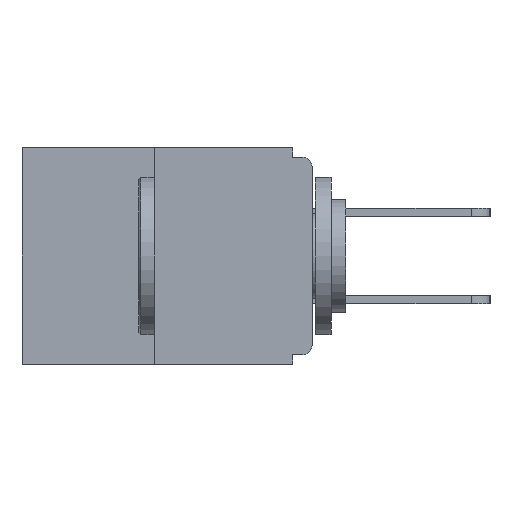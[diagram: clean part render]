
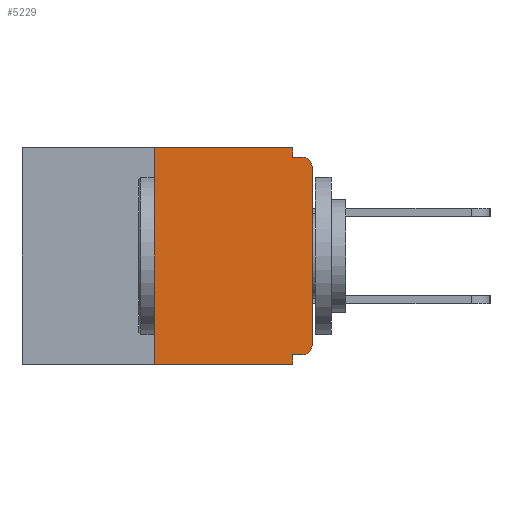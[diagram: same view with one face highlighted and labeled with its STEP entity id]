
A CAD part, left-side view. The second image highlights one B-rep face of the part: STEP entity #5229.
In plain terms, the highlighted planar face has unit normal (-1, 0, 0).
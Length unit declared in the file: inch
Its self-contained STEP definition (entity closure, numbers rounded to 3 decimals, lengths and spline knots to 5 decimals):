
#596 = AXIS2_PLACEMENT_3D ( 'NONE', #19665, #8271, #16163 ) ;
#840 = DIRECTION ( 'NONE',  ( 0., 0., -1. ) ) ;
#916 = ORIENTED_EDGE ( 'NONE', *, *, #10833, .F. ) ;
#1297 = DIRECTION ( 'NONE',  ( 0., 0., 1. ) ) ;
#1313 = PLANE ( 'NONE',  #23732 ) ;
#1740 = CARTESIAN_POINT ( 'NONE',  ( 0., 0., -0.328 ) ) ;
#2377 = FACE_OUTER_BOUND ( 'NONE', #3800, .T. ) ;
#2539 = DIRECTION ( 'NONE',  ( 0., 0., 1. ) ) ;
#3269 = CARTESIAN_POINT ( 'NONE',  ( 0., 0., -0.313 ) ) ;
#3676 = DIRECTION ( 'NONE',  ( 0., 0., -1. ) ) ;
#3800 = EDGE_LOOP ( 'NONE', ( #14801, #8469, #24225, #5966, #916, #23715, #18617, #8338, #15374, #19220 ) ) ;
#3841 = EDGE_CURVE ( 'NONE', #18358, #21685, #25170, .T. ) ;
#5088 = EDGE_CURVE ( 'NONE', #18833, #5514, #5436, .T. ) ;
#5229 = ADVANCED_FACE ( 'NONE', ( #2377 ), #1313, .F. ) ;
#5434 = CARTESIAN_POINT ( 'NONE',  ( 0., 0.015, -0.328 ) ) ;
#5436 = LINE ( 'NONE', #8785, #19596 ) ;
#5514 = VERTEX_POINT ( 'NONE', #10177 ) ;
#5833 = CARTESIAN_POINT ( 'NONE',  ( 0., 0.015, -0.03 ) ) ;
#5950 = VECTOR ( 'NONE', #2539, 39.37008 ) ;
#5966 = ORIENTED_EDGE ( 'NONE', *, *, #5088, .F. ) ;
#6164 = CARTESIAN_POINT ( 'NONE',  ( 0., 0.031, 0. ) ) ;
#6411 = CARTESIAN_POINT ( 'NONE',  ( 0., 0.015, -0.015 ) ) ;
#6547 = DIRECTION ( 'NONE',  ( 0., -1., 0. ) ) ;
#6632 = AXIS2_PLACEMENT_3D ( 'NONE', #5833, #23604, #3676 ) ;
#6744 = EDGE_CURVE ( 'NONE', #7429, #5514, #15855, .T. ) ;
#6960 = DIRECTION ( 'NONE',  ( 1., 0., 0. ) ) ;
#7358 = EDGE_CURVE ( 'NONE', #16632, #21954, #15472, .T. ) ;
#7429 = VERTEX_POINT ( 'NONE', #8364 ) ;
#8271 = DIRECTION ( 'NONE',  ( -1., 0., 0. ) ) ;
#8338 = ORIENTED_EDGE ( 'NONE', *, *, #22774, .T. ) ;
#8364 = CARTESIAN_POINT ( 'NONE',  ( 0., 0.25, -0.343 ) ) ;
#8469 = ORIENTED_EDGE ( 'NONE', *, *, #19182, .F. ) ;
#8528 = CARTESIAN_POINT ( 'NONE',  ( 0., 0.25, 0. ) ) ;
#8785 = CARTESIAN_POINT ( 'NONE',  ( 0., 0.031, -0.343 ) ) ;
#8950 = CARTESIAN_POINT ( 'NONE',  ( 0., 0.46, -0.343 ) ) ;
#10177 = CARTESIAN_POINT ( 'NONE',  ( 0., 0.031, -0.343 ) ) ;
#10534 = LINE ( 'NONE', #1740, #24949 ) ;
#10624 = CARTESIAN_POINT ( 'NONE',  ( 0., 0.031, 0. ) ) ;
#10833 = EDGE_CURVE ( 'NONE', #16566, #18833, #10534, .T. ) ;
#10983 = CARTESIAN_POINT ( 'NONE',  ( 0., 0.46, 0. ) ) ;
#12148 = VECTOR ( 'NONE', #13732, 39.37008 ) ;
#12721 = LINE ( 'NONE', #13194, #13337 ) ;
#12729 = DIRECTION ( 'NONE',  ( 0., -1., 0. ) ) ;
#13194 = CARTESIAN_POINT ( 'NONE',  ( 0., 0.25, 0. ) ) ;
#13337 = VECTOR ( 'NONE', #1297, 39.37008 ) ;
#13732 = DIRECTION ( 'NONE',  ( 0., -1., 0. ) ) ;
#14092 = DIRECTION ( 'NONE',  ( 0., 0., -1. ) ) ;
#14193 = VECTOR ( 'NONE', #6547, 39.37008 ) ;
#14526 = EDGE_CURVE ( 'NONE', #18059, #16936, #16650, .T. ) ;
#14801 = ORIENTED_EDGE ( 'NONE', *, *, #3841, .F. ) ;
#15374 = ORIENTED_EDGE ( 'NONE', *, *, #14526, .F. ) ;
#15472 = LINE ( 'NONE', #20176, #5950 ) ;
#15855 = LINE ( 'NONE', #8950, #12148 ) ;
#15954 = EDGE_CURVE ( 'NONE', #16566, #16632, #23313, .T. ) ;
#16163 = DIRECTION ( 'NONE',  ( 0., 0., -1. ) ) ;
#16566 = VERTEX_POINT ( 'NONE', #5434 ) ;
#16632 = VERTEX_POINT ( 'NONE', #3269 ) ;
#16650 = LINE ( 'NONE', #24216, #14193 ) ;
#16897 = VECTOR ( 'NONE', #12729, 39.37008 ) ;
#16936 = VERTEX_POINT ( 'NONE', #6411 ) ;
#17451 = CARTESIAN_POINT ( 'NONE',  ( 0., 0., -0.03 ) ) ;
#17682 = DIRECTION ( 'NONE',  ( 0., 1., 0. ) ) ;
#18059 = VERTEX_POINT ( 'NONE', #20958 ) ;
#18321 = CIRCLE ( 'NONE', #6632, 0.015 ) ;
#18358 = VERTEX_POINT ( 'NONE', #8528 ) ;
#18617 = ORIENTED_EDGE ( 'NONE', *, *, #7358, .T. ) ;
#18794 = DIRECTION ( 'NONE',  ( 0., 0., -1. ) ) ;
#18833 = VERTEX_POINT ( 'NONE', #19757 ) ;
#19182 = EDGE_CURVE ( 'NONE', #7429, #18358, #12721, .T. ) ;
#19220 = ORIENTED_EDGE ( 'NONE', *, *, #19343, .F. ) ;
#19343 = EDGE_CURVE ( 'NONE', #21685, #18059, #21331, .T. ) ;
#19596 = VECTOR ( 'NONE', #840, 39.37008 ) ;
#19665 = CARTESIAN_POINT ( 'NONE',  ( 0., 0.015, -0.313 ) ) ;
#19757 = CARTESIAN_POINT ( 'NONE',  ( 0., 0.031, -0.328 ) ) ;
#20176 = CARTESIAN_POINT ( 'NONE',  ( 0., 0., 0. ) ) ;
#20564 = CARTESIAN_POINT ( 'NONE',  ( 0., 0.46, 0. ) ) ;
#20958 = CARTESIAN_POINT ( 'NONE',  ( 0., 0.031, -0.015 ) ) ;
#21331 = LINE ( 'NONE', #6164, #24392 ) ;
#21685 = VERTEX_POINT ( 'NONE', #10624 ) ;
#21954 = VERTEX_POINT ( 'NONE', #17451 ) ;
#22774 = EDGE_CURVE ( 'NONE', #21954, #16936, #18321, .T. ) ;
#23313 = CIRCLE ( 'NONE', #596, 0.015 ) ;
#23604 = DIRECTION ( 'NONE',  ( -1., 0., 0. ) ) ;
#23715 = ORIENTED_EDGE ( 'NONE', *, *, #15954, .T. ) ;
#23732 = AXIS2_PLACEMENT_3D ( 'NONE', #10983, #6960, #18794 ) ;
#24216 = CARTESIAN_POINT ( 'NONE',  ( 0., 0., -0.015 ) ) ;
#24225 = ORIENTED_EDGE ( 'NONE', *, *, #6744, .T. ) ;
#24392 = VECTOR ( 'NONE', #14092, 39.37008 ) ;
#24949 = VECTOR ( 'NONE', #17682, 39.37008 ) ;
#25170 = LINE ( 'NONE', #20564, #16897 ) ;
